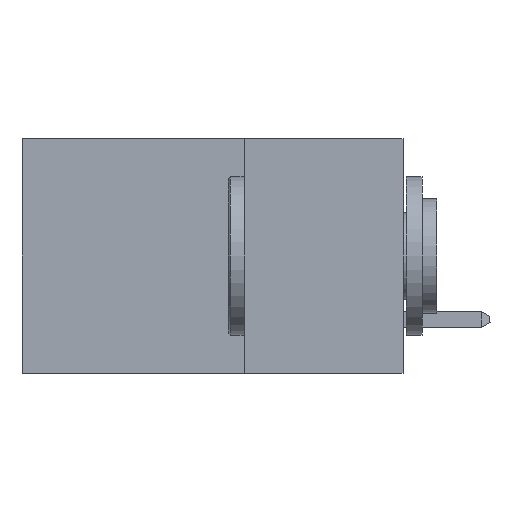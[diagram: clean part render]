
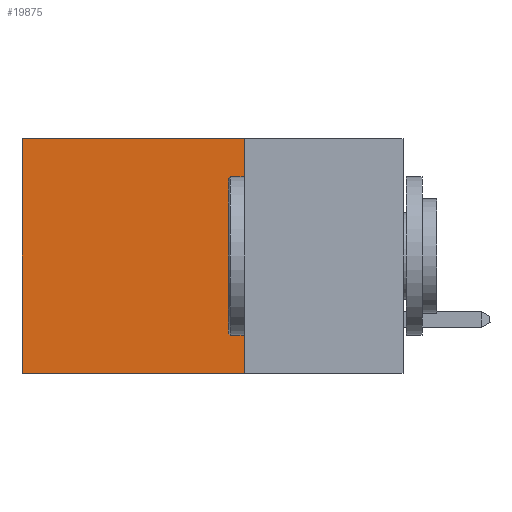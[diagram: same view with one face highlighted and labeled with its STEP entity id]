
A CAD part, left-side view. The second image highlights one B-rep face of the part: STEP entity #19875.
In plain terms, the highlighted planar face has unit normal (-1, 0, 0).
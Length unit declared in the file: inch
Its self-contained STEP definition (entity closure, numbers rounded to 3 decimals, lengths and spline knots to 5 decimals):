
#521 = ORIENTED_EDGE ( 'NONE', *, *, #771, .F. ) ;
#771 = EDGE_CURVE ( 'NONE', #21367, #8900, #27512, .T. ) ;
#992 = VECTOR ( 'NONE', #11451, 39.37008 ) ;
#1334 = VECTOR ( 'NONE', #6047, 39.37008 ) ;
#4247 = CARTESIAN_POINT ( 'NONE',  ( 0.2875, 0.25, 0. ) ) ;
#6047 = DIRECTION ( 'NONE',  ( 0., 1., 0. ) ) ;
#6227 = DIRECTION ( 'NONE',  ( 0., 0., -1. ) ) ;
#6429 = CARTESIAN_POINT ( 'NONE',  ( 0.2875, 0.25, 0. ) ) ;
#6771 = PLANE ( 'NONE',  #18931 ) ;
#7127 = LINE ( 'NONE', #27016, #992 ) ;
#8900 = VERTEX_POINT ( 'NONE', #13120 ) ;
#10267 = CARTESIAN_POINT ( 'NONE',  ( 0.2875, 0.6, 0. ) ) ;
#10550 = LINE ( 'NONE', #29080, #18858 ) ;
#11451 = DIRECTION ( 'NONE',  ( 0., 1., 0. ) ) ;
#12326 = VECTOR ( 'NONE', #6227, 39.37008 ) ;
#12429 = VERTEX_POINT ( 'NONE', #10267 ) ;
#12469 = CARTESIAN_POINT ( 'NONE',  ( 0.2875, 0.25, -0.37 ) ) ;
#12742 = DIRECTION ( 'NONE',  ( 0., 0., -1. ) ) ;
#13120 = CARTESIAN_POINT ( 'NONE',  ( 0.2875, 0.25, -0.37 ) ) ;
#14308 = FACE_OUTER_BOUND ( 'NONE', #17459, .T. ) ;
#15649 = DIRECTION ( 'NONE',  ( 1., 0., 0. ) ) ;
#17223 = CARTESIAN_POINT ( 'NONE',  ( 0.2875, 0.6, -0.37 ) ) ;
#17459 = EDGE_LOOP ( 'NONE', ( #18593, #26250, #521, #27892 ) ) ;
#18593 = ORIENTED_EDGE ( 'NONE', *, *, #23094, .T. ) ;
#18858 = VECTOR ( 'NONE', #12742, 39.37008 ) ;
#18931 = AXIS2_PLACEMENT_3D ( 'NONE', #4247, #15649, #20709 ) ;
#19838 = CARTESIAN_POINT ( 'NONE',  ( 0.2875, 0.25, 0. ) ) ;
#19875 = ADVANCED_FACE ( 'NONE', ( #14308 ), #6771, .F. ) ;
#20325 = EDGE_CURVE ( 'NONE', #8900, #22556, #28213, .T. ) ;
#20550 = EDGE_CURVE ( 'NONE', #21367, #12429, #7127, .T. ) ;
#20709 = DIRECTION ( 'NONE',  ( 0., 0., -1. ) ) ;
#21367 = VERTEX_POINT ( 'NONE', #19838 ) ;
#22556 = VERTEX_POINT ( 'NONE', #17223 ) ;
#23094 = EDGE_CURVE ( 'NONE', #12429, #22556, #10550, .T. ) ;
#26250 = ORIENTED_EDGE ( 'NONE', *, *, #20325, .F. ) ;
#27016 = CARTESIAN_POINT ( 'NONE',  ( 0.2875, 0.25, 0. ) ) ;
#27512 = LINE ( 'NONE', #6429, #12326 ) ;
#27892 = ORIENTED_EDGE ( 'NONE', *, *, #20550, .T. ) ;
#28213 = LINE ( 'NONE', #12469, #1334 ) ;
#29080 = CARTESIAN_POINT ( 'NONE',  ( 0.2875, 0.6, 0. ) ) ;
